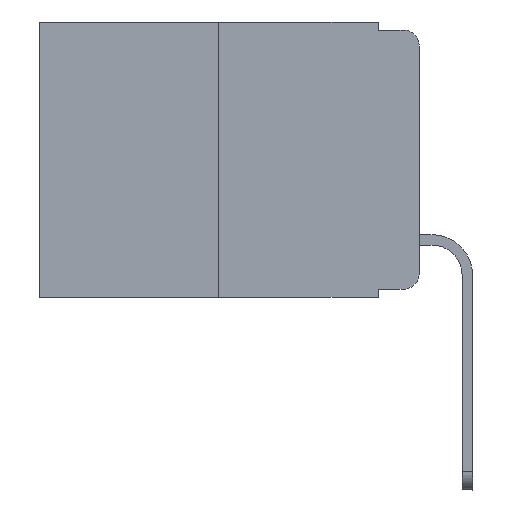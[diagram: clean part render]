
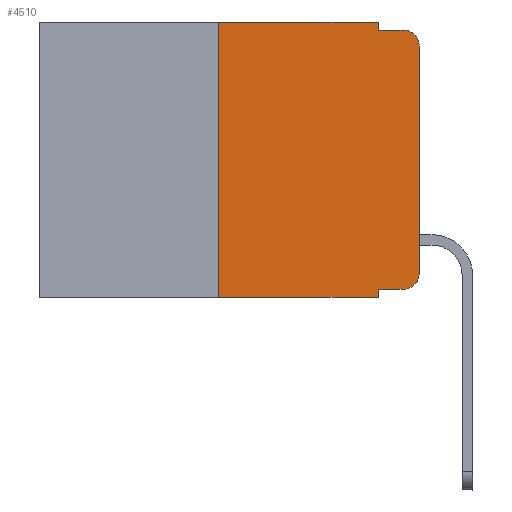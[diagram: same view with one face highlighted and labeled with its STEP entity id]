
A CAD part, left-side view. The second image highlights one B-rep face of the part: STEP entity #4510.
In plain terms, the highlighted planar face has unit normal (-1, 0, 0).
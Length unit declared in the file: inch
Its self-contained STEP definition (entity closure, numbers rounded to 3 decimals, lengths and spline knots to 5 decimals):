
#148 = EDGE_CURVE ( 'NONE', #11914, #3491, #8414, .T. ) ;
#174 = CARTESIAN_POINT ( 'NONE',  ( 0., 0.051, 0. ) ) ;
#317 = ORIENTED_EDGE ( 'NONE', *, *, #4829, .T. ) ;
#516 = DIRECTION ( 'NONE',  ( -1., 0., 0. ) ) ;
#556 = AXIS2_PLACEMENT_3D ( 'NONE', #4150, #6137, #8104 ) ;
#826 = ORIENTED_EDGE ( 'NONE', *, *, #8071, .F. ) ;
#918 = VECTOR ( 'NONE', #7458, 39.37008 ) ;
#950 = CIRCLE ( 'NONE', #556, 0.02 ) ;
#1087 = EDGE_CURVE ( 'NONE', #1140, #7621, #6454, .T. ) ;
#1140 = VERTEX_POINT ( 'NONE', #1278 ) ;
#1269 = CARTESIAN_POINT ( 'NONE',  ( 0., 0.02, -0.313 ) ) ;
#1271 = CARTESIAN_POINT ( 'NONE',  ( 0., 0.473, 0. ) ) ;
#1278 = CARTESIAN_POINT ( 'NONE',  ( 0., 0.051, -0.01 ) ) ;
#1369 = CARTESIAN_POINT ( 'NONE',  ( 0., 0.02, -0.01 ) ) ;
#1429 = VECTOR ( 'NONE', #12096, 39.37008 ) ;
#1485 = VERTEX_POINT ( 'NONE', #9608 ) ;
#1898 = CARTESIAN_POINT ( 'NONE',  ( 0., 0.473, -0.343 ) ) ;
#2064 = CARTESIAN_POINT ( 'NONE',  ( 0., 0.051, -0.333 ) ) ;
#2205 = VECTOR ( 'NONE', #11683, 39.37008 ) ;
#3130 = PLANE ( 'NONE',  #10718 ) ;
#3164 = CARTESIAN_POINT ( 'NONE',  ( 0., 0., 0. ) ) ;
#3277 = ORIENTED_EDGE ( 'NONE', *, *, #4642, .T. ) ;
#3344 = VERTEX_POINT ( 'NONE', #3686 ) ;
#3491 = VERTEX_POINT ( 'NONE', #174 ) ;
#3686 = CARTESIAN_POINT ( 'NONE',  ( 0., 0.25, -0.343 ) ) ;
#3876 = CARTESIAN_POINT ( 'NONE',  ( 0., 0.051, 0. ) ) ;
#4020 = CIRCLE ( 'NONE', #9620, 0.02 ) ;
#4047 = CARTESIAN_POINT ( 'NONE',  ( 0., 0.051, 0. ) ) ;
#4150 = CARTESIAN_POINT ( 'NONE',  ( 0., 0.02, -0.03 ) ) ;
#4170 = ORIENTED_EDGE ( 'NONE', *, *, #6488, .F. ) ;
#4294 = LINE ( 'NONE', #7109, #7181 ) ;
#4510 = ADVANCED_FACE ( 'NONE', ( #11709 ), #3130, .F. ) ;
#4530 = VECTOR ( 'NONE', #8946, 39.37008 ) ;
#4642 = EDGE_CURVE ( 'NONE', #3344, #12085, #5360, .T. ) ;
#4712 = CARTESIAN_POINT ( 'NONE',  ( 0., 0.25, 0. ) ) ;
#4829 = EDGE_CURVE ( 'NONE', #1485, #10093, #7945, .T. ) ;
#5182 = EDGE_CURVE ( 'NONE', #10387, #7621, #950, .T. ) ;
#5360 = LINE ( 'NONE', #1898, #6745 ) ;
#5371 = CARTESIAN_POINT ( 'NONE',  ( 0., 0.473, 0. ) ) ;
#6091 = ORIENTED_EDGE ( 'NONE', *, *, #6690, .T. ) ;
#6137 = DIRECTION ( 'NONE',  ( -1., 0., 0. ) ) ;
#6454 = LINE ( 'NONE', #11362, #1429 ) ;
#6488 = EDGE_CURVE ( 'NONE', #1485, #12085, #6552, .T. ) ;
#6552 = LINE ( 'NONE', #3876, #8383 ) ;
#6578 = CARTESIAN_POINT ( 'NONE',  ( 0., 0.02, -0.333 ) ) ;
#6690 = EDGE_CURVE ( 'NONE', #11180, #10387, #11736, .T. ) ;
#6745 = VECTOR ( 'NONE', #7707, 39.37008 ) ;
#6974 = DIRECTION ( 'NONE',  ( 0., 0., 1. ) ) ;
#7109 = CARTESIAN_POINT ( 'NONE',  ( 0., 0.25, 0. ) ) ;
#7150 = CARTESIAN_POINT ( 'NONE',  ( 0., 0.051, -0.343 ) ) ;
#7181 = VECTOR ( 'NONE', #12059, 39.37008 ) ;
#7188 = DIRECTION ( 'NONE',  ( 0., 0., -1. ) ) ;
#7458 = DIRECTION ( 'NONE',  ( 0., -1., 0. ) ) ;
#7497 = EDGE_LOOP ( 'NONE', ( #6091, #11993, #10527, #826, #8429, #9346, #3277, #4170, #317, #11714 ) ) ;
#7621 = VERTEX_POINT ( 'NONE', #1369 ) ;
#7707 = DIRECTION ( 'NONE',  ( 0., -1., 0. ) ) ;
#7745 = LINE ( 'NONE', #4047, #2205 ) ;
#7781 = EDGE_CURVE ( 'NONE', #3344, #11914, #4294, .T. ) ;
#7945 = LINE ( 'NONE', #2064, #4530 ) ;
#8021 = CARTESIAN_POINT ( 'NONE',  ( 0., 0., -0.03 ) ) ;
#8071 = EDGE_CURVE ( 'NONE', #3491, #1140, #7745, .T. ) ;
#8104 = DIRECTION ( 'NONE',  ( 0., 0., -1. ) ) ;
#8181 = VECTOR ( 'NONE', #6974, 39.37008 ) ;
#8383 = VECTOR ( 'NONE', #10398, 39.37008 ) ;
#8414 = LINE ( 'NONE', #5371, #918 ) ;
#8429 = ORIENTED_EDGE ( 'NONE', *, *, #148, .F. ) ;
#8946 = DIRECTION ( 'NONE',  ( 0., -1., 0. ) ) ;
#9084 = EDGE_CURVE ( 'NONE', #10093, #11180, #4020, .T. ) ;
#9346 = ORIENTED_EDGE ( 'NONE', *, *, #7781, .F. ) ;
#9608 = CARTESIAN_POINT ( 'NONE',  ( 0., 0.051, -0.333 ) ) ;
#9620 = AXIS2_PLACEMENT_3D ( 'NONE', #1269, #516, #7188 ) ;
#10093 = VERTEX_POINT ( 'NONE', #6578 ) ;
#10204 = DIRECTION ( 'NONE',  ( 0., 0., -1. ) ) ;
#10387 = VERTEX_POINT ( 'NONE', #8021 ) ;
#10398 = DIRECTION ( 'NONE',  ( 0., 0., -1. ) ) ;
#10527 = ORIENTED_EDGE ( 'NONE', *, *, #1087, .F. ) ;
#10718 = AXIS2_PLACEMENT_3D ( 'NONE', #1271, #12074, #10204 ) ;
#10864 = CARTESIAN_POINT ( 'NONE',  ( 0., 0., -0.313 ) ) ;
#11180 = VERTEX_POINT ( 'NONE', #10864 ) ;
#11362 = CARTESIAN_POINT ( 'NONE',  ( 0., 0.051, -0.01 ) ) ;
#11683 = DIRECTION ( 'NONE',  ( 0., 0., -1. ) ) ;
#11709 = FACE_OUTER_BOUND ( 'NONE', #7497, .T. ) ;
#11714 = ORIENTED_EDGE ( 'NONE', *, *, #9084, .T. ) ;
#11736 = LINE ( 'NONE', #3164, #8181 ) ;
#11914 = VERTEX_POINT ( 'NONE', #4712 ) ;
#11993 = ORIENTED_EDGE ( 'NONE', *, *, #5182, .T. ) ;
#12059 = DIRECTION ( 'NONE',  ( 0., 0., 1. ) ) ;
#12074 = DIRECTION ( 'NONE',  ( 1., 0., 0. ) ) ;
#12085 = VERTEX_POINT ( 'NONE', #7150 ) ;
#12096 = DIRECTION ( 'NONE',  ( 0., -1., 0. ) ) ;
